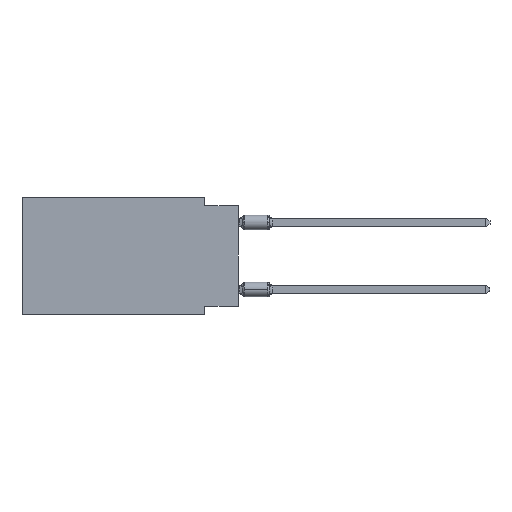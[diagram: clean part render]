
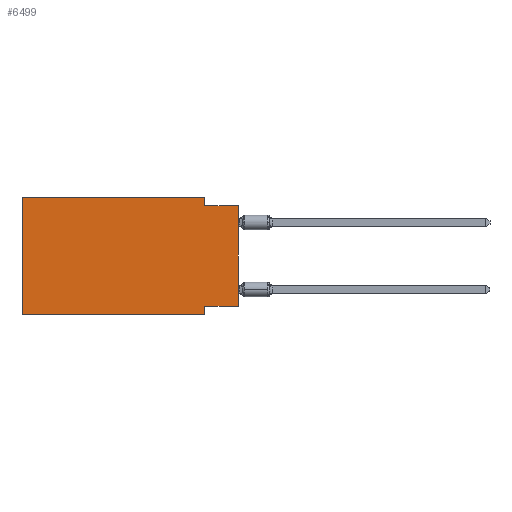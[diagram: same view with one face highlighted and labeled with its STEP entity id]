
A CAD part, left-side view. The second image highlights one B-rep face of the part: STEP entity #6499.
In plain terms, the highlighted planar face has unit normal (-1, 0, 0).
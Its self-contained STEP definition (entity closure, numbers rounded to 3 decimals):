
#58 = FACE_OUTER_BOUND ( 'NONE', #10982, .T. ) ;
#105 = LINE ( 'NONE', #4272, #12140 ) ;
#168 = CARTESIAN_POINT ( 'NONE',  ( 0., 16.383, -8.89 ) ) ;
#321 = ORIENTED_EDGE ( 'NONE', *, *, #11486, .F. ) ;
#478 = VERTEX_POINT ( 'NONE', #3950 ) ;
#598 = VERTEX_POINT ( 'NONE', #5243 ) ;
#745 = DIRECTION ( 'NONE',  ( 0., -1., 0. ) ) ;
#760 = LINE ( 'NONE', #8812, #6121 ) ;
#786 = DIRECTION ( 'NONE',  ( 0., 0., -1. ) ) ;
#860 = ORIENTED_EDGE ( 'NONE', *, *, #12999, .T. ) ;
#1061 = DIRECTION ( 'NONE',  ( 0., -1., 0. ) ) ;
#1570 = ORIENTED_EDGE ( 'NONE', *, *, #4047, .T. ) ;
#2213 = VECTOR ( 'NONE', #1061, 1000. ) ;
#2665 = VECTOR ( 'NONE', #10672, 1000. ) ;
#3004 = CARTESIAN_POINT ( 'NONE',  ( 0., 16.383, 0. ) ) ;
#3221 = CARTESIAN_POINT ( 'NONE',  ( 0., 0., -8.255 ) ) ;
#3256 = EDGE_CURVE ( 'NONE', #598, #6632, #105, .T. ) ;
#3376 = CARTESIAN_POINT ( 'NONE',  ( 0., 2.54, 0. ) ) ;
#3950 = CARTESIAN_POINT ( 'NONE',  ( 0., 0., -0.635 ) ) ;
#4015 = CARTESIAN_POINT ( 'NONE',  ( 0., 16.383, 0. ) ) ;
#4023 = PLANE ( 'NONE',  #4970 ) ;
#4047 = EDGE_CURVE ( 'NONE', #598, #12821, #12454, .T. ) ;
#4104 = VECTOR ( 'NONE', #745, 1000. ) ;
#4125 = EDGE_CURVE ( 'NONE', #7388, #11817, #9310, .T. ) ;
#4131 = VERTEX_POINT ( 'NONE', #5638 ) ;
#4272 = CARTESIAN_POINT ( 'NONE',  ( 0., 16.383, 0. ) ) ;
#4970 = AXIS2_PLACEMENT_3D ( 'NONE', #3004, #11381, #12278 ) ;
#5243 = CARTESIAN_POINT ( 'NONE',  ( 0., 16.383, -8.89 ) ) ;
#5398 = CARTESIAN_POINT ( 'NONE',  ( 0., 0., 0. ) ) ;
#5638 = CARTESIAN_POINT ( 'NONE',  ( 0., 2.54, -8.255 ) ) ;
#6121 = VECTOR ( 'NONE', #9081, 1000. ) ;
#6499 = ADVANCED_FACE ( 'NONE', ( #58 ), #4023, .F. ) ;
#6632 = VERTEX_POINT ( 'NONE', #9741 ) ;
#7388 = VERTEX_POINT ( 'NONE', #11180 ) ;
#7434 = EDGE_CURVE ( 'NONE', #6632, #7388, #9192, .T. ) ;
#7812 = CARTESIAN_POINT ( 'NONE',  ( 0., 0., -0.635 ) ) ;
#8154 = CARTESIAN_POINT ( 'NONE',  ( 0., 2.54, -0.635 ) ) ;
#8525 = EDGE_CURVE ( 'NONE', #4131, #12821, #10071, .T. ) ;
#8658 = LINE ( 'NONE', #5398, #11672 ) ;
#8687 = LINE ( 'NONE', #7812, #9948 ) ;
#8772 = EDGE_CURVE ( 'NONE', #11817, #478, #8687, .T. ) ;
#8812 = CARTESIAN_POINT ( 'NONE',  ( 0., 0., -8.255 ) ) ;
#9081 = DIRECTION ( 'NONE',  ( 0., 1., 0. ) ) ;
#9124 = VERTEX_POINT ( 'NONE', #3221 ) ;
#9192 = LINE ( 'NONE', #4015, #4104 ) ;
#9310 = LINE ( 'NONE', #3376, #2665 ) ;
#9741 = CARTESIAN_POINT ( 'NONE',  ( 0., 16.383, 0. ) ) ;
#9754 = DIRECTION ( 'NONE',  ( 0., 0., 1. ) ) ;
#9948 = VECTOR ( 'NONE', #10803, 1000. ) ;
#10071 = LINE ( 'NONE', #12381, #11252 ) ;
#10493 = ORIENTED_EDGE ( 'NONE', *, *, #4125, .F. ) ;
#10672 = DIRECTION ( 'NONE',  ( 0., 0., -1. ) ) ;
#10803 = DIRECTION ( 'NONE',  ( 0., -1., 0. ) ) ;
#10918 = ORIENTED_EDGE ( 'NONE', *, *, #8525, .F. ) ;
#10982 = EDGE_LOOP ( 'NONE', ( #860, #11535, #10493, #11413, #11485, #1570, #10918, #321 ) ) ;
#11180 = CARTESIAN_POINT ( 'NONE',  ( 0., 2.54, 0. ) ) ;
#11252 = VECTOR ( 'NONE', #786, 1000. ) ;
#11361 = DIRECTION ( 'NONE',  ( 0., 0., 1. ) ) ;
#11381 = DIRECTION ( 'NONE',  ( 1., 0., 0. ) ) ;
#11413 = ORIENTED_EDGE ( 'NONE', *, *, #7434, .F. ) ;
#11485 = ORIENTED_EDGE ( 'NONE', *, *, #3256, .F. ) ;
#11486 = EDGE_CURVE ( 'NONE', #9124, #4131, #760, .T. ) ;
#11527 = CARTESIAN_POINT ( 'NONE',  ( 0., 2.54, -8.89 ) ) ;
#11535 = ORIENTED_EDGE ( 'NONE', *, *, #8772, .F. ) ;
#11672 = VECTOR ( 'NONE', #9754, 1000. ) ;
#11817 = VERTEX_POINT ( 'NONE', #8154 ) ;
#12140 = VECTOR ( 'NONE', #11361, 1000. ) ;
#12278 = DIRECTION ( 'NONE',  ( 0., 0., -1. ) ) ;
#12381 = CARTESIAN_POINT ( 'NONE',  ( 0., 2.54, -8.89 ) ) ;
#12454 = LINE ( 'NONE', #168, #2213 ) ;
#12821 = VERTEX_POINT ( 'NONE', #11527 ) ;
#12999 = EDGE_CURVE ( 'NONE', #9124, #478, #8658, .T. ) ;
